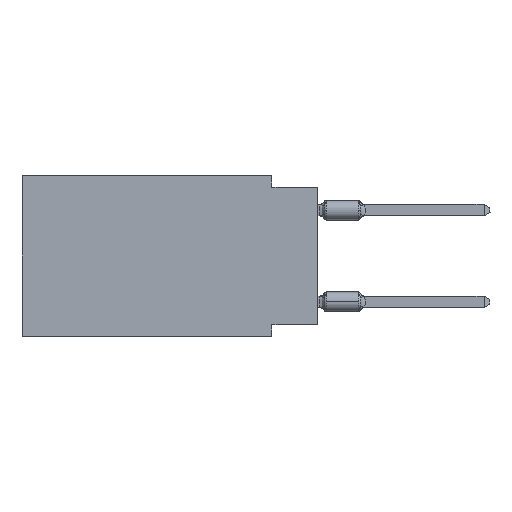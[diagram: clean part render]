
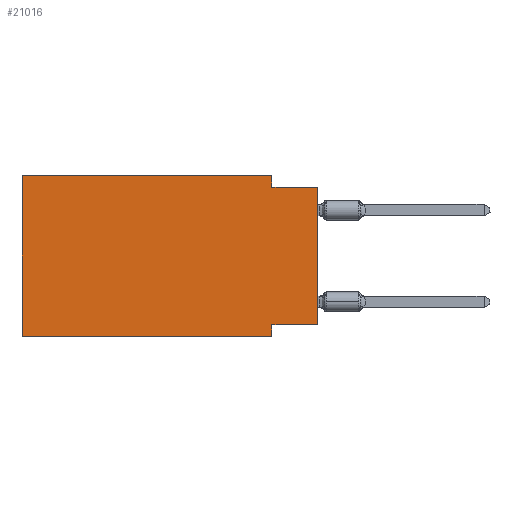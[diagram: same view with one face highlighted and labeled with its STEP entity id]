
A CAD part, left-side view. The second image highlights one B-rep face of the part: STEP entity #21016.
In plain terms, the highlighted planar face has unit normal (-1, 0, 0).
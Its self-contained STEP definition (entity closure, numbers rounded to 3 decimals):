
#668 = VERTEX_POINT ( 'NONE', #36846 ) ;
#815 = VECTOR ( 'NONE', #11111, 1000. ) ;
#880 = EDGE_CURVE ( 'NONE', #35489, #56238, #52898, .T. ) ;
#2758 = CARTESIAN_POINT ( 'NONE',  ( 0., 2.54, -8.89 ) ) ;
#2760 = CARTESIAN_POINT ( 'NONE',  ( 0., 0., -8.255 ) ) ;
#3914 = CARTESIAN_POINT ( 'NONE',  ( 0., 16.383, 0. ) ) ;
#6298 = LINE ( 'NONE', #19207, #44063 ) ;
#7631 = CARTESIAN_POINT ( 'NONE',  ( 0., 2.54, 0. ) ) ;
#9190 = FACE_OUTER_BOUND ( 'NONE', #20604, .T. ) ;
#9462 = CARTESIAN_POINT ( 'NONE',  ( 0., 0., -0.635 ) ) ;
#10819 = CARTESIAN_POINT ( 'NONE',  ( 0., 0., -0.635 ) ) ;
#10829 = CARTESIAN_POINT ( 'NONE',  ( 0., 16.383, -8.89 ) ) ;
#11111 = DIRECTION ( 'NONE',  ( 0., -1., 0. ) ) ;
#12986 = ORIENTED_EDGE ( 'NONE', *, *, #56306, .F. ) ;
#13524 = DIRECTION ( 'NONE',  ( 0., 0., 1. ) ) ;
#15682 = LINE ( 'NONE', #7631, #47683 ) ;
#16887 = ORIENTED_EDGE ( 'NONE', *, *, #28529, .F. ) ;
#17801 = CARTESIAN_POINT ( 'NONE',  ( 0., 16.383, 0. ) ) ;
#19207 = CARTESIAN_POINT ( 'NONE',  ( 0., 2.54, -8.89 ) ) ;
#19802 = DIRECTION ( 'NONE',  ( 0., 0., -1. ) ) ;
#20604 = EDGE_LOOP ( 'NONE', ( #40166, #26192, #55143, #16887, #50414, #40673, #12986, #31240 ) ) ;
#21016 = ADVANCED_FACE ( 'NONE', ( #9190 ), #30733, .F. ) ;
#21097 = DIRECTION ( 'NONE',  ( 0., 0., -1. ) ) ;
#21307 = VECTOR ( 'NONE', #37791, 1000. ) ;
#24843 = AXIS2_PLACEMENT_3D ( 'NONE', #53711, #41631, #19802 ) ;
#25424 = LINE ( 'NONE', #2760, #21307 ) ;
#26192 = ORIENTED_EDGE ( 'NONE', *, *, #50467, .F. ) ;
#26745 = CARTESIAN_POINT ( 'NONE',  ( 0., 0., 0. ) ) ;
#27349 = CARTESIAN_POINT ( 'NONE',  ( 0., 2.54, -8.255 ) ) ;
#28342 = DIRECTION ( 'NONE',  ( 0., -1., 0. ) ) ;
#28529 = EDGE_CURVE ( 'NONE', #56191, #668, #29772, .T. ) ;
#28991 = DIRECTION ( 'NONE',  ( 0., 0., -1. ) ) ;
#29772 = LINE ( 'NONE', #3914, #36692 ) ;
#29875 = LINE ( 'NONE', #47667, #33720 ) ;
#30733 = PLANE ( 'NONE',  #24843 ) ;
#31240 = ORIENTED_EDGE ( 'NONE', *, *, #38076, .F. ) ;
#31283 = VERTEX_POINT ( 'NONE', #2758 ) ;
#33518 = DIRECTION ( 'NONE',  ( 0., -1., 0. ) ) ;
#33720 = VECTOR ( 'NONE', #34730, 1000. ) ;
#34517 = EDGE_CURVE ( 'NONE', #668, #50691, #15682, .T. ) ;
#34730 = DIRECTION ( 'NONE',  ( 0., 0., 1. ) ) ;
#35489 = VERTEX_POINT ( 'NONE', #56524 ) ;
#36412 = VECTOR ( 'NONE', #28342, 1000. ) ;
#36692 = VECTOR ( 'NONE', #33518, 1000. ) ;
#36846 = CARTESIAN_POINT ( 'NONE',  ( 0., 2.54, 0. ) ) ;
#36936 = LINE ( 'NONE', #10819, #36412 ) ;
#37791 = DIRECTION ( 'NONE',  ( 0., 1., 0. ) ) ;
#37812 = VECTOR ( 'NONE', #13524, 1000. ) ;
#38076 = EDGE_CURVE ( 'NONE', #35489, #55631, #25424, .T. ) ;
#40166 = ORIENTED_EDGE ( 'NONE', *, *, #880, .T. ) ;
#40673 = ORIENTED_EDGE ( 'NONE', *, *, #54889, .T. ) ;
#41631 = DIRECTION ( 'NONE',  ( 1., 0., 0. ) ) ;
#42297 = CARTESIAN_POINT ( 'NONE',  ( 0., 16.383, -8.89 ) ) ;
#42939 = VERTEX_POINT ( 'NONE', #42297 ) ;
#44063 = VECTOR ( 'NONE', #28991, 1000. ) ;
#47667 = CARTESIAN_POINT ( 'NONE',  ( 0., 16.383, 0. ) ) ;
#47683 = VECTOR ( 'NONE', #21097, 1000. ) ;
#48385 = CARTESIAN_POINT ( 'NONE',  ( 0., 2.54, -0.635 ) ) ;
#50168 = LINE ( 'NONE', #10829, #815 ) ;
#50414 = ORIENTED_EDGE ( 'NONE', *, *, #53025, .F. ) ;
#50467 = EDGE_CURVE ( 'NONE', #50691, #56238, #36936, .T. ) ;
#50691 = VERTEX_POINT ( 'NONE', #48385 ) ;
#52898 = LINE ( 'NONE', #26745, #37812 ) ;
#53025 = EDGE_CURVE ( 'NONE', #42939, #56191, #29875, .T. ) ;
#53711 = CARTESIAN_POINT ( 'NONE',  ( 0., 16.383, 0. ) ) ;
#54889 = EDGE_CURVE ( 'NONE', #42939, #31283, #50168, .T. ) ;
#55143 = ORIENTED_EDGE ( 'NONE', *, *, #34517, .F. ) ;
#55631 = VERTEX_POINT ( 'NONE', #27349 ) ;
#56191 = VERTEX_POINT ( 'NONE', #17801 ) ;
#56238 = VERTEX_POINT ( 'NONE', #9462 ) ;
#56306 = EDGE_CURVE ( 'NONE', #55631, #31283, #6298, .T. ) ;
#56524 = CARTESIAN_POINT ( 'NONE',  ( 0., 0., -8.255 ) ) ;
